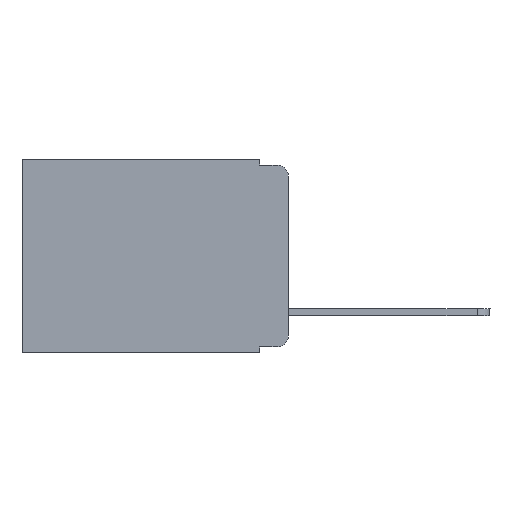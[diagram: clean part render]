
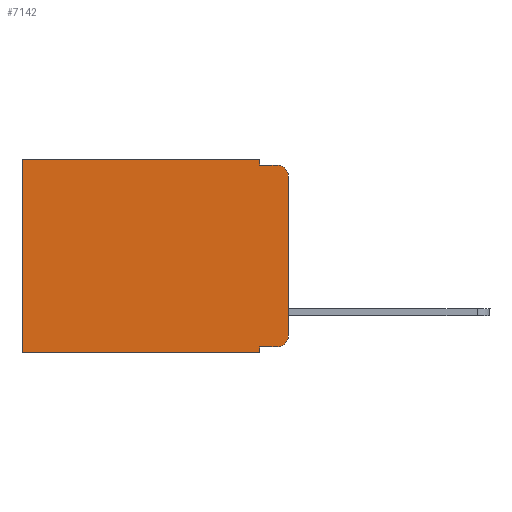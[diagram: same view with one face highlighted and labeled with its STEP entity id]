
A CAD part, left-side view. The second image highlights one B-rep face of the part: STEP entity #7142.
In plain terms, the highlighted planar face has unit normal (-1, 0, 0).
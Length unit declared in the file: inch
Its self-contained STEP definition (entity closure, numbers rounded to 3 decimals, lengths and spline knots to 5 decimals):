
#110 = LINE ( 'NONE', #3557, #4154 ) ;
#179 = CARTESIAN_POINT ( 'NONE',  ( 0.298, 0., 0. ) ) ;
#704 = VECTOR ( 'NONE', #9497, 39.37008 ) ;
#761 = VECTOR ( 'NONE', #3489, 39.37008 ) ;
#765 = VECTOR ( 'NONE', #7901, 39.37008 ) ;
#899 = EDGE_CURVE ( 'NONE', #8551, #10883, #13373, .T. ) ;
#1041 = EDGE_CURVE ( 'NONE', #10852, #5214, #14133, .T. ) ;
#1105 = LINE ( 'NONE', #13983, #15101 ) ;
#1130 = DIRECTION ( 'NONE',  ( 0., 0., -1. ) ) ;
#1632 = EDGE_CURVE ( 'NONE', #5214, #10883, #110, .T. ) ;
#1813 = DIRECTION ( 'NONE',  ( 0., 0., -1. ) ) ;
#1866 = CARTESIAN_POINT ( 'NONE',  ( 0.298, 0.02, -0.01 ) ) ;
#2285 = CARTESIAN_POINT ( 'NONE',  ( 0.298, 0.02, -0.03 ) ) ;
#2473 = PLANE ( 'NONE',  #5160 ) ;
#2733 = CARTESIAN_POINT ( 'NONE',  ( 0.298, 0.473, -0.343 ) ) ;
#3061 = ORIENTED_EDGE ( 'NONE', *, *, #7792, .F. ) ;
#3200 = CIRCLE ( 'NONE', #5641, 0.02 ) ;
#3489 = DIRECTION ( 'NONE',  ( 0., -1., 0. ) ) ;
#3557 = CARTESIAN_POINT ( 'NONE',  ( 0.298, 0.473, 0. ) ) ;
#3705 = EDGE_LOOP ( 'NONE', ( #9656, #9528, #3061, #12808, #11482, #10025, #6110, #10749, #13715, #11122 ) ) ;
#3956 = VECTOR ( 'NONE', #4849, 39.37008 ) ;
#4146 = VERTEX_POINT ( 'NONE', #9774 ) ;
#4154 = VECTOR ( 'NONE', #9537, 39.37008 ) ;
#4430 = CARTESIAN_POINT ( 'NONE',  ( 0.298, 0., -0.03 ) ) ;
#4534 = DIRECTION ( 'NONE',  ( 0., 0., -1. ) ) ;
#4849 = DIRECTION ( 'NONE',  ( 0., 0., -1. ) ) ;
#4961 = LINE ( 'NONE', #9645, #704 ) ;
#5160 = AXIS2_PLACEMENT_3D ( 'NONE', #10894, #13201, #7342 ) ;
#5193 = VERTEX_POINT ( 'NONE', #1866 ) ;
#5205 = VECTOR ( 'NONE', #9610, 39.37008 ) ;
#5214 = VERTEX_POINT ( 'NONE', #5380 ) ;
#5380 = CARTESIAN_POINT ( 'NONE',  ( 0.298, 0.473, 0. ) ) ;
#5533 = CARTESIAN_POINT ( 'NONE',  ( 0.298, 0., -0.343 ) ) ;
#5641 = AXIS2_PLACEMENT_3D ( 'NONE', #2285, #5868, #1130 ) ;
#5868 = DIRECTION ( 'NONE',  ( -1., 0., 0. ) ) ;
#6110 = ORIENTED_EDGE ( 'NONE', *, *, #899, .F. ) ;
#6354 = CARTESIAN_POINT ( 'NONE',  ( 0.298, 0.051, -0.343 ) ) ;
#6417 = DIRECTION ( 'NONE',  ( 0., -1., 0. ) ) ;
#6482 = CARTESIAN_POINT ( 'NONE',  ( 0.298, 0., -0.313 ) ) ;
#6652 = EDGE_CURVE ( 'NONE', #4146, #9760, #13994, .T. ) ;
#7142 = ADVANCED_FACE ( 'NONE', ( #8496 ), #2473, .F. ) ;
#7342 = DIRECTION ( 'NONE',  ( 0., 0., -1. ) ) ;
#7433 = CARTESIAN_POINT ( 'NONE',  ( 0.298, 0.051, -0.01 ) ) ;
#7538 = CARTESIAN_POINT ( 'NONE',  ( 0.298, 0.02, -0.313 ) ) ;
#7541 = LINE ( 'NONE', #12251, #10778 ) ;
#7792 = EDGE_CURVE ( 'NONE', #11440, #5193, #7541, .T. ) ;
#7901 = DIRECTION ( 'NONE',  ( 0., 1., 0. ) ) ;
#7999 = EDGE_CURVE ( 'NONE', #10332, #5193, #3200, .T. ) ;
#8206 = CARTESIAN_POINT ( 'NONE',  ( 0.298, 0.051, -0.333 ) ) ;
#8496 = FACE_OUTER_BOUND ( 'NONE', #3705, .T. ) ;
#8551 = VERTEX_POINT ( 'NONE', #6354 ) ;
#8875 = EDGE_CURVE ( 'NONE', #4146, #8551, #4961, .T. ) ;
#9031 = CIRCLE ( 'NONE', #12973, 0.02 ) ;
#9312 = EDGE_CURVE ( 'NONE', #9760, #11894, #9031, .T. ) ;
#9497 = DIRECTION ( 'NONE',  ( 0., 0., -1. ) ) ;
#9528 = ORIENTED_EDGE ( 'NONE', *, *, #7999, .T. ) ;
#9537 = DIRECTION ( 'NONE',  ( 0., 0., -1. ) ) ;
#9610 = DIRECTION ( 'NONE',  ( 0., 1., 0. ) ) ;
#9645 = CARTESIAN_POINT ( 'NONE',  ( 0.298, 0.051, 0. ) ) ;
#9656 = ORIENTED_EDGE ( 'NONE', *, *, #13558, .F. ) ;
#9760 = VERTEX_POINT ( 'NONE', #14803 ) ;
#9774 = CARTESIAN_POINT ( 'NONE',  ( 0.298, 0.051, -0.333 ) ) ;
#10025 = ORIENTED_EDGE ( 'NONE', *, *, #1632, .T. ) ;
#10332 = VERTEX_POINT ( 'NONE', #4430 ) ;
#10749 = ORIENTED_EDGE ( 'NONE', *, *, #8875, .F. ) ;
#10778 = VECTOR ( 'NONE', #6417, 39.37008 ) ;
#10852 = VERTEX_POINT ( 'NONE', #14309 ) ;
#10883 = VERTEX_POINT ( 'NONE', #2733 ) ;
#10894 = CARTESIAN_POINT ( 'NONE',  ( 0.298, 0., 0. ) ) ;
#11122 = ORIENTED_EDGE ( 'NONE', *, *, #9312, .T. ) ;
#11440 = VERTEX_POINT ( 'NONE', #7433 ) ;
#11482 = ORIENTED_EDGE ( 'NONE', *, *, #1041, .T. ) ;
#11853 = LINE ( 'NONE', #179, #3956 ) ;
#11894 = VERTEX_POINT ( 'NONE', #6482 ) ;
#12246 = DIRECTION ( 'NONE',  ( -1., 0., 0. ) ) ;
#12251 = CARTESIAN_POINT ( 'NONE',  ( 0.298, 0.051, -0.01 ) ) ;
#12808 = ORIENTED_EDGE ( 'NONE', *, *, #15055, .F. ) ;
#12973 = AXIS2_PLACEMENT_3D ( 'NONE', #7538, #12246, #1813 ) ;
#13201 = DIRECTION ( 'NONE',  ( 1., 0., 0. ) ) ;
#13373 = LINE ( 'NONE', #5533, #765 ) ;
#13558 = EDGE_CURVE ( 'NONE', #10332, #11894, #11853, .T. ) ;
#13715 = ORIENTED_EDGE ( 'NONE', *, *, #6652, .T. ) ;
#13983 = CARTESIAN_POINT ( 'NONE',  ( 0.298, 0.051, 0. ) ) ;
#13994 = LINE ( 'NONE', #8206, #761 ) ;
#14133 = LINE ( 'NONE', #14289, #5205 ) ;
#14289 = CARTESIAN_POINT ( 'NONE',  ( 0.298, 0., 0. ) ) ;
#14309 = CARTESIAN_POINT ( 'NONE',  ( 0.298, 0.051, 0. ) ) ;
#14803 = CARTESIAN_POINT ( 'NONE',  ( 0.298, 0.02, -0.333 ) ) ;
#15055 = EDGE_CURVE ( 'NONE', #10852, #11440, #1105, .T. ) ;
#15101 = VECTOR ( 'NONE', #4534, 39.37008 ) ;
